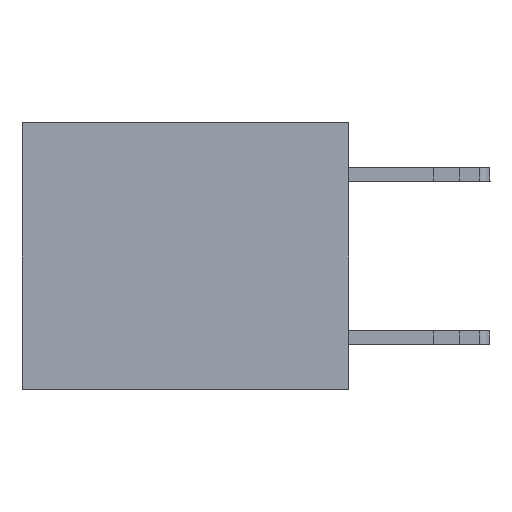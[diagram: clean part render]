
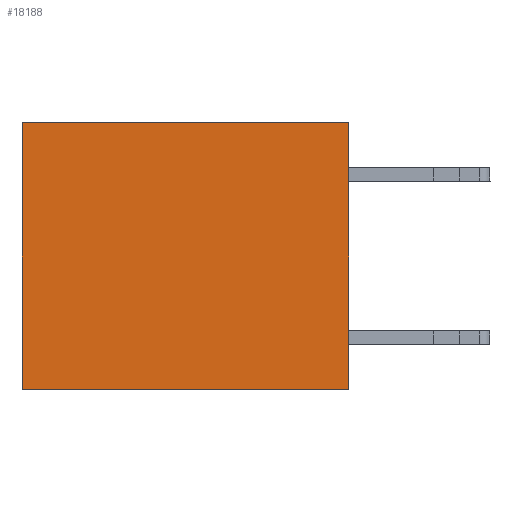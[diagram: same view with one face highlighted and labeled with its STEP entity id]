
A CAD part, left-side view. The second image highlights one B-rep face of the part: STEP entity #18188.
In plain terms, the highlighted planar face has unit normal (-1, 0, 0).
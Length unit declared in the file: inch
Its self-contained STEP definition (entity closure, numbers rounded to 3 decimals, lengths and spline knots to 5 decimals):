
#107 = VERTEX_POINT ( 'NONE', #13988 ) ;
#3180 = EDGE_CURVE ( 'NONE', #107, #17128, #10047, .T. ) ;
#3201 = DIRECTION ( 'NONE',  ( 0., 0., -1. ) ) ;
#3593 = CARTESIAN_POINT ( 'NONE',  ( 0.3165, 0., 0. ) ) ;
#4605 = VECTOR ( 'NONE', #10100, 39.37008 ) ;
#5554 = DIRECTION ( 'NONE',  ( 1., 0., 0. ) ) ;
#5617 = EDGE_CURVE ( 'NONE', #9866, #17128, #17860, .T. ) ;
#8573 = LINE ( 'NONE', #3593, #8911 ) ;
#8739 = EDGE_LOOP ( 'NONE', ( #16163, #27125, #17763, #16447 ) ) ;
#8911 = VECTOR ( 'NONE', #24829, 39.37008 ) ;
#9477 = AXIS2_PLACEMENT_3D ( 'NONE', #9855, #5554, #3201 ) ;
#9855 = CARTESIAN_POINT ( 'NONE',  ( 0.3165, 0., -0.49 ) ) ;
#9866 = VERTEX_POINT ( 'NONE', #24729 ) ;
#10047 = LINE ( 'NONE', #10628, #10389 ) ;
#10100 = DIRECTION ( 'NONE',  ( 0., 0., -1. ) ) ;
#10389 = VECTOR ( 'NONE', #16604, 39.37008 ) ;
#10628 = CARTESIAN_POINT ( 'NONE',  ( 0.3165, 0.6, -0.49 ) ) ;
#11305 = LINE ( 'NONE', #14205, #4605 ) ;
#12399 = EDGE_CURVE ( 'NONE', #22730, #9866, #11305, .T. ) ;
#12948 = EDGE_CURVE ( 'NONE', #22730, #107, #8573, .T. ) ;
#13988 = CARTESIAN_POINT ( 'NONE',  ( 0.3165, 0.6, 0. ) ) ;
#14205 = CARTESIAN_POINT ( 'NONE',  ( 0.3165, 0., -0.49 ) ) ;
#14958 = CARTESIAN_POINT ( 'NONE',  ( 0.3165, 0., -0.49 ) ) ;
#16049 = CARTESIAN_POINT ( 'NONE',  ( 0.3165, 0., 0. ) ) ;
#16108 = PLANE ( 'NONE',  #9477 ) ;
#16163 = ORIENTED_EDGE ( 'NONE', *, *, #3180, .T. ) ;
#16447 = ORIENTED_EDGE ( 'NONE', *, *, #12948, .T. ) ;
#16604 = DIRECTION ( 'NONE',  ( 0., 0., -1. ) ) ;
#17128 = VERTEX_POINT ( 'NONE', #27187 ) ;
#17172 = VECTOR ( 'NONE', #19149, 39.37008 ) ;
#17763 = ORIENTED_EDGE ( 'NONE', *, *, #12399, .F. ) ;
#17860 = LINE ( 'NONE', #14958, #17172 ) ;
#18188 = ADVANCED_FACE ( 'NONE', ( #22632 ), #16108, .F. ) ;
#19149 = DIRECTION ( 'NONE',  ( 0., 1., 0. ) ) ;
#22632 = FACE_OUTER_BOUND ( 'NONE', #8739, .T. ) ;
#22730 = VERTEX_POINT ( 'NONE', #16049 ) ;
#24729 = CARTESIAN_POINT ( 'NONE',  ( 0.3165, 0., -0.49 ) ) ;
#24829 = DIRECTION ( 'NONE',  ( 0., 1., 0. ) ) ;
#27125 = ORIENTED_EDGE ( 'NONE', *, *, #5617, .F. ) ;
#27187 = CARTESIAN_POINT ( 'NONE',  ( 0.3165, 0.6, -0.49 ) ) ;
